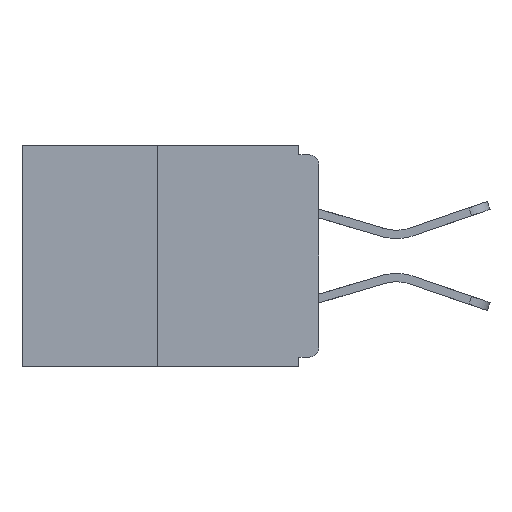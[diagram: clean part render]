
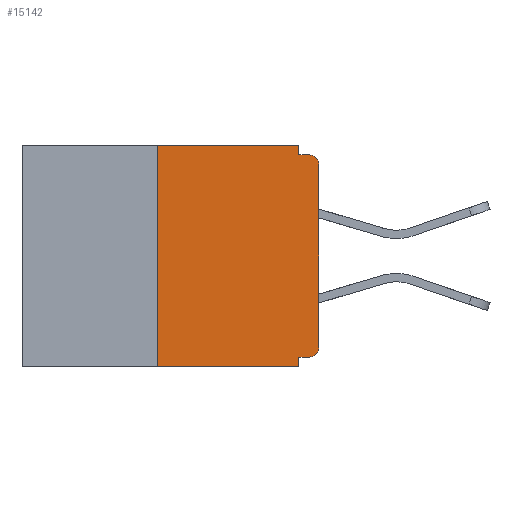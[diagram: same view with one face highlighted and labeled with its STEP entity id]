
A CAD part, left-side view. The second image highlights one B-rep face of the part: STEP entity #15142.
In plain terms, the highlighted planar face has unit normal (-1, 0, 0).
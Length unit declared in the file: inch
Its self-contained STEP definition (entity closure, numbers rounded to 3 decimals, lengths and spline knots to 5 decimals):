
#295 = AXIS2_PLACEMENT_3D ( 'NONE', #9991, #2474, #22935 ) ;
#449 = LINE ( 'NONE', #10746, #19279 ) ;
#1784 = CARTESIAN_POINT ( 'NONE',  ( 0., 0., -0.015 ) ) ;
#2474 = DIRECTION ( 'NONE',  ( -1., 0., 0. ) ) ;
#2631 = LINE ( 'NONE', #8169, #14507 ) ;
#2778 = CARTESIAN_POINT ( 'NONE',  ( 0., 0., -0.328 ) ) ;
#2958 = CARTESIAN_POINT ( 'NONE',  ( 0., 0.031, -0.015 ) ) ;
#3930 = DIRECTION ( 'NONE',  ( 1., 0., 0. ) ) ;
#4050 = EDGE_CURVE ( 'NONE', #17954, #17231, #8632, .T. ) ;
#4478 = VERTEX_POINT ( 'NONE', #2958 ) ;
#4726 = DIRECTION ( 'NONE',  ( 0., 0., -1. ) ) ;
#5067 = ORIENTED_EDGE ( 'NONE', *, *, #21312, .F. ) ;
#5152 = EDGE_CURVE ( 'NONE', #13456, #14374, #18150, .T. ) ;
#5636 = VECTOR ( 'NONE', #6023, 39.37008 ) ;
#5873 = VECTOR ( 'NONE', #19954, 39.37008 ) ;
#5968 = VECTOR ( 'NONE', #12416, 39.37008 ) ;
#6023 = DIRECTION ( 'NONE',  ( 0., -1., 0. ) ) ;
#6605 = CARTESIAN_POINT ( 'NONE',  ( 0., 0.015, -0.03 ) ) ;
#6827 = ORIENTED_EDGE ( 'NONE', *, *, #22928, .F. ) ;
#6988 = VERTEX_POINT ( 'NONE', #12442 ) ;
#7221 = CARTESIAN_POINT ( 'NONE',  ( 0., 0., 0. ) ) ;
#7653 = CIRCLE ( 'NONE', #295, 0.015 ) ;
#7955 = ORIENTED_EDGE ( 'NONE', *, *, #10137, .F. ) ;
#7991 = CARTESIAN_POINT ( 'NONE',  ( 0., 0.015, -0.328 ) ) ;
#8169 = CARTESIAN_POINT ( 'NONE',  ( 0., 0.031, 0. ) ) ;
#8310 = ORIENTED_EDGE ( 'NONE', *, *, #4050, .T. ) ;
#8478 = CARTESIAN_POINT ( 'NONE',  ( 0., 0.25, 0. ) ) ;
#8632 = CIRCLE ( 'NONE', #18293, 0.015 ) ;
#8722 = LINE ( 'NONE', #7221, #9898 ) ;
#9217 = DIRECTION ( 'NONE',  ( 0., -1., 0. ) ) ;
#9898 = VECTOR ( 'NONE', #16231, 39.37008 ) ;
#9915 = EDGE_CURVE ( 'NONE', #13456, #6988, #449, .T. ) ;
#9991 = CARTESIAN_POINT ( 'NONE',  ( 0., 0.015, -0.313 ) ) ;
#10137 = EDGE_CURVE ( 'NONE', #14374, #13176, #12601, .T. ) ;
#10143 = CARTESIAN_POINT ( 'NONE',  ( 0., 0.015, -0.015 ) ) ;
#10203 = EDGE_CURVE ( 'NONE', #10839, #22745, #7653, .T. ) ;
#10534 = CARTESIAN_POINT ( 'NONE',  ( 0., 0.031, 0. ) ) ;
#10610 = ORIENTED_EDGE ( 'NONE', *, *, #19767, .F. ) ;
#10746 = CARTESIAN_POINT ( 'NONE',  ( 0., 0.46, -0.343 ) ) ;
#10839 = VERTEX_POINT ( 'NONE', #7991 ) ;
#11224 = DIRECTION ( 'NONE',  ( 0., -1., 0. ) ) ;
#11492 = VECTOR ( 'NONE', #23826, 39.37008 ) ;
#11682 = AXIS2_PLACEMENT_3D ( 'NONE', #20559, #3930, #18768 ) ;
#12416 = DIRECTION ( 'NONE',  ( 0., 0., 1. ) ) ;
#12442 = CARTESIAN_POINT ( 'NONE',  ( 0., 0.031, -0.343 ) ) ;
#12601 = LINE ( 'NONE', #15102, #5636 ) ;
#13176 = VERTEX_POINT ( 'NONE', #10534 ) ;
#13456 = VERTEX_POINT ( 'NONE', #21291 ) ;
#13947 = DIRECTION ( 'NONE',  ( 0., 0., -1. ) ) ;
#14374 = VERTEX_POINT ( 'NONE', #8478 ) ;
#14507 = VECTOR ( 'NONE', #13947, 39.37008 ) ;
#15045 = PLANE ( 'NONE',  #11682 ) ;
#15102 = CARTESIAN_POINT ( 'NONE',  ( 0., 0.46, 0. ) ) ;
#15142 = ADVANCED_FACE ( 'NONE', ( #18897 ), #15045, .F. ) ;
#15575 = ORIENTED_EDGE ( 'NONE', *, *, #22240, .T. ) ;
#16231 = DIRECTION ( 'NONE',  ( 0., 0., 1. ) ) ;
#16293 = EDGE_LOOP ( 'NONE', ( #7955, #22978, #22171, #10610, #5067, #21556, #15575, #8310, #6827, #22060 ) ) ;
#16296 = CARTESIAN_POINT ( 'NONE',  ( 0., 0.25, 0. ) ) ;
#16538 = CARTESIAN_POINT ( 'NONE',  ( 0., 0.031, -0.343 ) ) ;
#17231 = VERTEX_POINT ( 'NONE', #10143 ) ;
#17954 = VERTEX_POINT ( 'NONE', #19230 ) ;
#18150 = LINE ( 'NONE', #16296, #5968 ) ;
#18293 = AXIS2_PLACEMENT_3D ( 'NONE', #6605, #19488, #4726 ) ;
#18417 = LINE ( 'NONE', #16538, #11492 ) ;
#18768 = DIRECTION ( 'NONE',  ( 0., 0., -1. ) ) ;
#18897 = FACE_OUTER_BOUND ( 'NONE', #16293, .T. ) ;
#19230 = CARTESIAN_POINT ( 'NONE',  ( 0., 0., -0.03 ) ) ;
#19279 = VECTOR ( 'NONE', #11224, 39.37008 ) ;
#19488 = DIRECTION ( 'NONE',  ( -1., 0., 0. ) ) ;
#19696 = LINE ( 'NONE', #1784, #20898 ) ;
#19767 = EDGE_CURVE ( 'NONE', #21819, #6988, #18417, .T. ) ;
#19954 = DIRECTION ( 'NONE',  ( 0., 1., 0. ) ) ;
#20559 = CARTESIAN_POINT ( 'NONE',  ( 0., 0.46, 0. ) ) ;
#20898 = VECTOR ( 'NONE', #9217, 39.37008 ) ;
#21291 = CARTESIAN_POINT ( 'NONE',  ( 0., 0.25, -0.343 ) ) ;
#21312 = EDGE_CURVE ( 'NONE', #10839, #21819, #23553, .T. ) ;
#21483 = CARTESIAN_POINT ( 'NONE',  ( 0., 0., -0.313 ) ) ;
#21556 = ORIENTED_EDGE ( 'NONE', *, *, #10203, .T. ) ;
#21819 = VERTEX_POINT ( 'NONE', #21971 ) ;
#21971 = CARTESIAN_POINT ( 'NONE',  ( 0., 0.031, -0.328 ) ) ;
#22060 = ORIENTED_EDGE ( 'NONE', *, *, #22625, .F. ) ;
#22171 = ORIENTED_EDGE ( 'NONE', *, *, #9915, .T. ) ;
#22240 = EDGE_CURVE ( 'NONE', #22745, #17954, #8722, .T. ) ;
#22625 = EDGE_CURVE ( 'NONE', #13176, #4478, #2631, .T. ) ;
#22745 = VERTEX_POINT ( 'NONE', #21483 ) ;
#22928 = EDGE_CURVE ( 'NONE', #4478, #17231, #19696, .T. ) ;
#22935 = DIRECTION ( 'NONE',  ( 0., 0., -1. ) ) ;
#22978 = ORIENTED_EDGE ( 'NONE', *, *, #5152, .F. ) ;
#23553 = LINE ( 'NONE', #2778, #5873 ) ;
#23826 = DIRECTION ( 'NONE',  ( 0., 0., -1. ) ) ;
